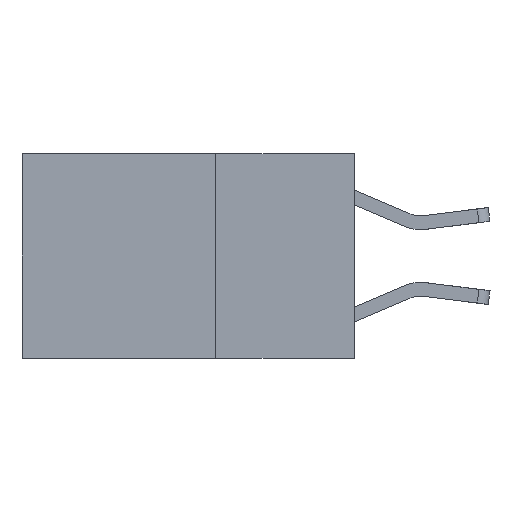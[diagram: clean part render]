
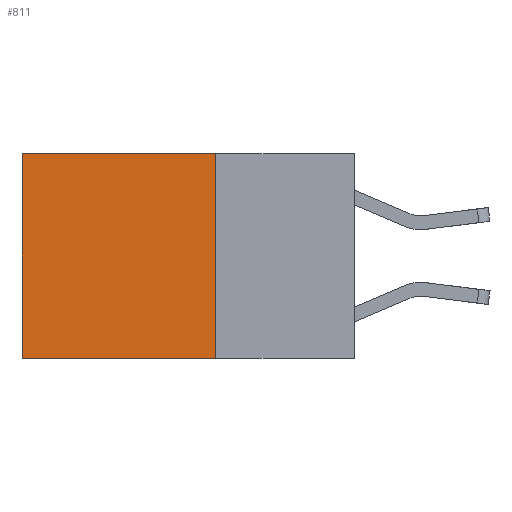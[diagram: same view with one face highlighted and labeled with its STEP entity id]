
A CAD part, left-side view. The second image highlights one B-rep face of the part: STEP entity #811.
In plain terms, the highlighted planar face has unit normal (-1, 0, 0).
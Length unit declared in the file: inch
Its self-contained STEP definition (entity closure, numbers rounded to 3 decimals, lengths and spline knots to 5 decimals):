
#251 = DIRECTION ( 'NONE',  ( 0., 0., -1. ) ) ;
#293 = DIRECTION ( 'NONE',  ( 1., 0., 0. ) ) ;
#389 = PLANE ( 'NONE',  #1123 ) ;
#461 = CARTESIAN_POINT ( 'NONE',  ( 0.2625, 0.25, 0. ) ) ;
#548 = DIRECTION ( 'NONE',  ( 0., 0., -1. ) ) ;
#575 = ORIENTED_EDGE ( 'NONE', *, *, #9963, .F. ) ;
#672 = VECTOR ( 'NONE', #1087, 39.37008 ) ;
#738 = CARTESIAN_POINT ( 'NONE',  ( 0.2625, 0.6, 0. ) ) ;
#811 = ADVANCED_FACE ( 'NONE', ( #7753 ), #389, .F. ) ;
#1087 = DIRECTION ( 'NONE',  ( 0., 0., -1. ) ) ;
#1123 = AXIS2_PLACEMENT_3D ( 'NONE', #461, #293, #251 ) ;
#1583 = CARTESIAN_POINT ( 'NONE',  ( 0.2625, 0.25, -0.37 ) ) ;
#1614 = LINE ( 'NONE', #9579, #7901 ) ;
#3040 = VERTEX_POINT ( 'NONE', #6971 ) ;
#3073 = VERTEX_POINT ( 'NONE', #738 ) ;
#3096 = VECTOR ( 'NONE', #8497, 39.37008 ) ;
#3586 = LINE ( 'NONE', #6935, #3096 ) ;
#3739 = VERTEX_POINT ( 'NONE', #1583 ) ;
#4077 = DIRECTION ( 'NONE',  ( 0., 1., 0. ) ) ;
#4224 = EDGE_CURVE ( 'NONE', #3739, #8188, #3586, .T. ) ;
#4469 = CARTESIAN_POINT ( 'NONE',  ( 0.2625, 0.6, 0. ) ) ;
#5741 = LINE ( 'NONE', #4469, #9926 ) ;
#5793 = EDGE_CURVE ( 'NONE', #3040, #3073, #1614, .T. ) ;
#6872 = EDGE_LOOP ( 'NONE', ( #7426, #9406, #575, #7154 ) ) ;
#6935 = CARTESIAN_POINT ( 'NONE',  ( 0.2625, 0.25, -0.37 ) ) ;
#6971 = CARTESIAN_POINT ( 'NONE',  ( 0.2625, 0.25, 0. ) ) ;
#7154 = ORIENTED_EDGE ( 'NONE', *, *, #5793, .T. ) ;
#7237 = EDGE_CURVE ( 'NONE', #3073, #8188, #5741, .T. ) ;
#7426 = ORIENTED_EDGE ( 'NONE', *, *, #7237, .T. ) ;
#7753 = FACE_OUTER_BOUND ( 'NONE', #6872, .T. ) ;
#7901 = VECTOR ( 'NONE', #4077, 39.37008 ) ;
#7976 = CARTESIAN_POINT ( 'NONE',  ( 0.2625, 0.6, -0.37 ) ) ;
#8142 = CARTESIAN_POINT ( 'NONE',  ( 0.2625, 0.25, 0. ) ) ;
#8188 = VERTEX_POINT ( 'NONE', #7976 ) ;
#8497 = DIRECTION ( 'NONE',  ( 0., 1., 0. ) ) ;
#9272 = LINE ( 'NONE', #8142, #672 ) ;
#9406 = ORIENTED_EDGE ( 'NONE', *, *, #4224, .F. ) ;
#9579 = CARTESIAN_POINT ( 'NONE',  ( 0.2625, 0.25, 0. ) ) ;
#9926 = VECTOR ( 'NONE', #548, 39.37008 ) ;
#9963 = EDGE_CURVE ( 'NONE', #3040, #3739, #9272, .T. ) ;
